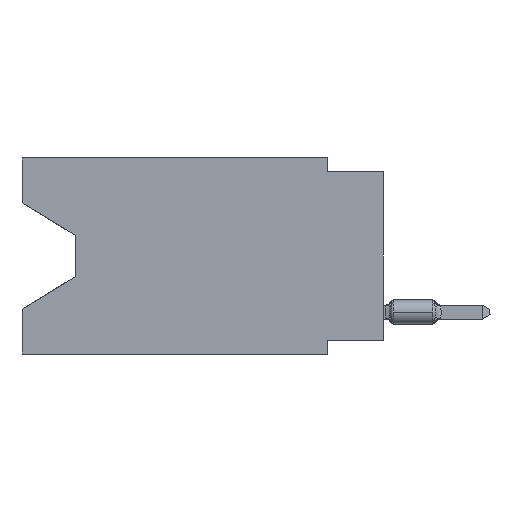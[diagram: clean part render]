
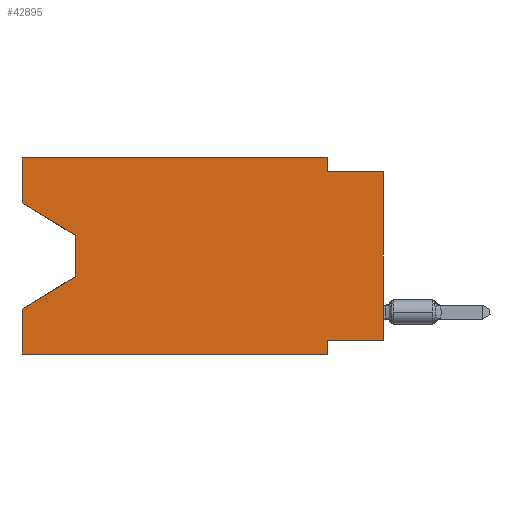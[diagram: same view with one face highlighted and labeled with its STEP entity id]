
A CAD part, left-side view. The second image highlights one B-rep face of the part: STEP entity #42895.
In plain terms, the highlighted planar face has unit normal (-1, 0, 0).
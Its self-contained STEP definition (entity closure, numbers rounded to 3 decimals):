
#557 = VECTOR ( 'NONE', #45963, 1000. ) ;
#559 = EDGE_CURVE ( 'NONE', #18016, #1429, #43694, .T. ) ;
#1429 = VERTEX_POINT ( 'NONE', #11151 ) ;
#2179 = CARTESIAN_POINT ( 'NONE',  ( 0., 16.383, 0. ) ) ;
#2632 = AXIS2_PLACEMENT_3D ( 'NONE', #48473, #5463, #13005 ) ;
#2848 = LINE ( 'NONE', #23064, #9409 ) ;
#2885 = CARTESIAN_POINT ( 'NONE',  ( 0., 13.97, -5.385 ) ) ;
#3972 = CARTESIAN_POINT ( 'NONE',  ( 0., 0., -8.255 ) ) ;
#4098 = CARTESIAN_POINT ( 'NONE',  ( 0., 16.383, 0. ) ) ;
#5159 = EDGE_CURVE ( 'NONE', #30214, #18358, #45063, .T. ) ;
#5463 = DIRECTION ( 'NONE',  ( 1., 0., 0. ) ) ;
#6025 = VECTOR ( 'NONE', #19924, 1000. ) ;
#6045 = LINE ( 'NONE', #49053, #35392 ) ;
#6466 = CARTESIAN_POINT ( 'NONE',  ( 0., 0., 0. ) ) ;
#8447 = CARTESIAN_POINT ( 'NONE',  ( 0., 16.383, -8.89 ) ) ;
#9409 = VECTOR ( 'NONE', #23312, 1000. ) ;
#9833 = DIRECTION ( 'NONE',  ( 0., 1., 0. ) ) ;
#9934 = DIRECTION ( 'NONE',  ( 0., 0.855, -0.519 ) ) ;
#9993 = DIRECTION ( 'NONE',  ( 0., 0., -1. ) ) ;
#10929 = VECTOR ( 'NONE', #33145, 1000. ) ;
#11151 = CARTESIAN_POINT ( 'NONE',  ( 0., 2.54, -8.89 ) ) ;
#11258 = ORIENTED_EDGE ( 'NONE', *, *, #29805, .F. ) ;
#12106 = VECTOR ( 'NONE', #45848, 1000. ) ;
#12384 = CARTESIAN_POINT ( 'NONE',  ( 0., 16.383, 0. ) ) ;
#12511 = EDGE_CURVE ( 'NONE', #47793, #1429, #48601, .T. ) ;
#12649 = CARTESIAN_POINT ( 'NONE',  ( 0., 2.54, 0. ) ) ;
#13005 = DIRECTION ( 'NONE',  ( 0., 0., -1. ) ) ;
#13015 = EDGE_LOOP ( 'NONE', ( #50835, #41995, #16538, #41331, #26521, #18765, #11258, #48196, #29709, #49020, #14303, #20752 ) ) ;
#13466 = LINE ( 'NONE', #29251, #30568 ) ;
#13666 = CARTESIAN_POINT ( 'NONE',  ( 0., 13.97, -3.505 ) ) ;
#13698 = VECTOR ( 'NONE', #39594, 1000. ) ;
#13984 = CARTESIAN_POINT ( 'NONE',  ( 0., 16.383, -2.038 ) ) ;
#14115 = LINE ( 'NONE', #2179, #557 ) ;
#14303 = ORIENTED_EDGE ( 'NONE', *, *, #40523, .F. ) ;
#15652 = LINE ( 'NONE', #46046, #35452 ) ;
#16538 = ORIENTED_EDGE ( 'NONE', *, *, #45882, .T. ) ;
#17073 = LINE ( 'NONE', #4098, #6025 ) ;
#17988 = EDGE_CURVE ( 'NONE', #29205, #39590, #15652, .T. ) ;
#18016 = VERTEX_POINT ( 'NONE', #47230 ) ;
#18358 = VERTEX_POINT ( 'NONE', #2885 ) ;
#18765 = ORIENTED_EDGE ( 'NONE', *, *, #12511, .F. ) ;
#19924 = DIRECTION ( 'NONE',  ( 0., 0., 1. ) ) ;
#20330 = EDGE_CURVE ( 'NONE', #29738, #37966, #17073, .T. ) ;
#20619 = VERTEX_POINT ( 'NONE', #3972 ) ;
#20752 = ORIENTED_EDGE ( 'NONE', *, *, #20330, .F. ) ;
#20960 = LINE ( 'NONE', #33643, #26489 ) ;
#23064 = CARTESIAN_POINT ( 'NONE',  ( 0., 16.383, -2.038 ) ) ;
#23312 = DIRECTION ( 'NONE',  ( 0., -0.855, -0.519 ) ) ;
#25162 = FACE_OUTER_BOUND ( 'NONE', #13015, .T. ) ;
#25871 = EDGE_CURVE ( 'NONE', #20619, #48572, #42212, .T. ) ;
#26489 = VECTOR ( 'NONE', #40413, 1000. ) ;
#26521 = ORIENTED_EDGE ( 'NONE', *, *, #559, .T. ) ;
#29205 = VERTEX_POINT ( 'NONE', #12649 ) ;
#29251 = CARTESIAN_POINT ( 'NONE',  ( 0., 0., -8.255 ) ) ;
#29709 = ORIENTED_EDGE ( 'NONE', *, *, #46116, .F. ) ;
#29738 = VERTEX_POINT ( 'NONE', #13984 ) ;
#29805 = EDGE_CURVE ( 'NONE', #20619, #47793, #13466, .T. ) ;
#30214 = VERTEX_POINT ( 'NONE', #13666 ) ;
#30568 = VECTOR ( 'NONE', #9833, 1000. ) ;
#32351 = EDGE_CURVE ( 'NONE', #18016, #33568, #14115, .T. ) ;
#32887 = CARTESIAN_POINT ( 'NONE',  ( 0., 2.54, -8.255 ) ) ;
#33145 = DIRECTION ( 'NONE',  ( 0., 0., -1. ) ) ;
#33568 = VERTEX_POINT ( 'NONE', #46012 ) ;
#33643 = CARTESIAN_POINT ( 'NONE',  ( 0., 0., -0.635 ) ) ;
#35392 = VECTOR ( 'NONE', #9934, 1000. ) ;
#35452 = VECTOR ( 'NONE', #37519, 1000. ) ;
#35554 = CARTESIAN_POINT ( 'NONE',  ( 0., 2.54, -0.635 ) ) ;
#36896 = VECTOR ( 'NONE', #9993, 1000. ) ;
#37044 = CARTESIAN_POINT ( 'NONE',  ( 0., 13.97, -3.505 ) ) ;
#37519 = DIRECTION ( 'NONE',  ( 0., 0., -1. ) ) ;
#37966 = VERTEX_POINT ( 'NONE', #47717 ) ;
#39590 = VERTEX_POINT ( 'NONE', #35554 ) ;
#39594 = DIRECTION ( 'NONE',  ( 0., -1., 0. ) ) ;
#40413 = DIRECTION ( 'NONE',  ( 0., -1., 0. ) ) ;
#40523 = EDGE_CURVE ( 'NONE', #37966, #29205, #47858, .T. ) ;
#40968 = PLANE ( 'NONE',  #2632 ) ;
#41098 = CARTESIAN_POINT ( 'NONE',  ( 0., 2.54, -8.89 ) ) ;
#41331 = ORIENTED_EDGE ( 'NONE', *, *, #32351, .F. ) ;
#41995 = ORIENTED_EDGE ( 'NONE', *, *, #5159, .T. ) ;
#42212 = LINE ( 'NONE', #6466, #12106 ) ;
#42744 = VECTOR ( 'NONE', #44206, 1000. ) ;
#42895 = ADVANCED_FACE ( 'NONE', ( #25162 ), #40968, .F. ) ;
#43694 = LINE ( 'NONE', #8447, #42744 ) ;
#44206 = DIRECTION ( 'NONE',  ( 0., -1., 0. ) ) ;
#45063 = LINE ( 'NONE', #37044, #10929 ) ;
#45848 = DIRECTION ( 'NONE',  ( 0., 0., 1. ) ) ;
#45882 = EDGE_CURVE ( 'NONE', #18358, #33568, #6045, .T. ) ;
#45963 = DIRECTION ( 'NONE',  ( 0., 0., 1. ) ) ;
#46012 = CARTESIAN_POINT ( 'NONE',  ( 0., 16.383, -6.852 ) ) ;
#46046 = CARTESIAN_POINT ( 'NONE',  ( 0., 2.54, 0. ) ) ;
#46116 = EDGE_CURVE ( 'NONE', #39590, #48572, #20960, .T. ) ;
#47230 = CARTESIAN_POINT ( 'NONE',  ( 0., 16.383, -8.89 ) ) ;
#47633 = EDGE_CURVE ( 'NONE', #29738, #30214, #2848, .T. ) ;
#47717 = CARTESIAN_POINT ( 'NONE',  ( 0., 16.383, 0. ) ) ;
#47793 = VERTEX_POINT ( 'NONE', #32887 ) ;
#47858 = LINE ( 'NONE', #12384, #13698 ) ;
#48196 = ORIENTED_EDGE ( 'NONE', *, *, #25871, .T. ) ;
#48473 = CARTESIAN_POINT ( 'NONE',  ( 0., 16.383, 0. ) ) ;
#48572 = VERTEX_POINT ( 'NONE', #50568 ) ;
#48601 = LINE ( 'NONE', #41098, #36896 ) ;
#49020 = ORIENTED_EDGE ( 'NONE', *, *, #17988, .F. ) ;
#49053 = CARTESIAN_POINT ( 'NONE',  ( 0., 13.97, -5.385 ) ) ;
#50568 = CARTESIAN_POINT ( 'NONE',  ( 0., 0., -0.635 ) ) ;
#50835 = ORIENTED_EDGE ( 'NONE', *, *, #47633, .T. ) ;
